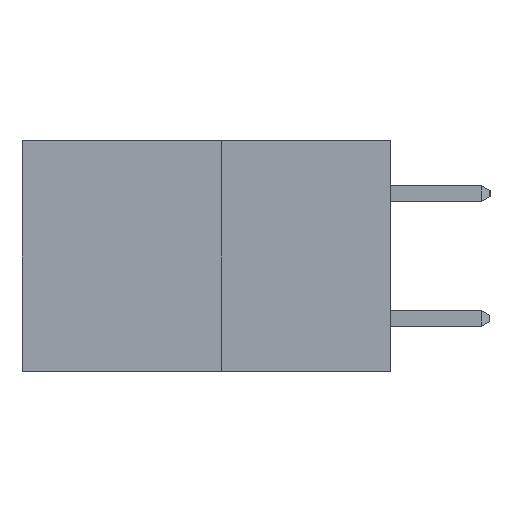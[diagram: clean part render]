
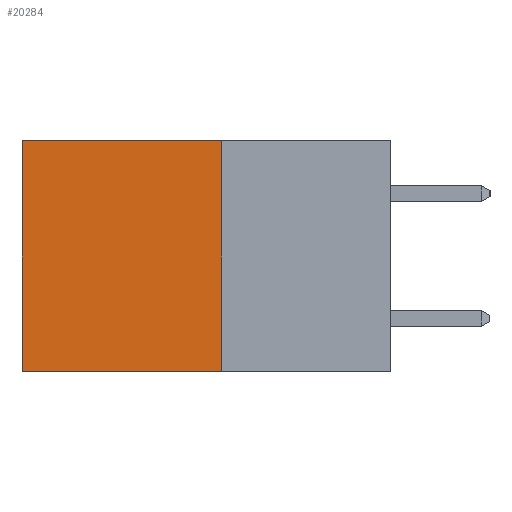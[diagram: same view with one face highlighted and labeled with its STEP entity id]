
A CAD part, left-side view. The second image highlights one B-rep face of the part: STEP entity #20284.
In plain terms, the highlighted planar face has unit normal (-1, 0, 0).
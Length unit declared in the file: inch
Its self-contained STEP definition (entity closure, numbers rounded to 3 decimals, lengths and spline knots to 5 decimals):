
#7 = CARTESIAN_POINT ( 'NONE',  ( 0.277, 0.59, 0. ) ) ;
#1687 = EDGE_CURVE ( 'NONE', #20280, #17652, #16281, .T. ) ;
#2284 = DIRECTION ( 'NONE',  ( 0., 0., -1. ) ) ;
#3063 = PLANE ( 'NONE',  #10664 ) ;
#3429 = VECTOR ( 'NONE', #18031, 39.37008 ) ;
#5241 = ORIENTED_EDGE ( 'NONE', *, *, #1687, .T. ) ;
#5421 = CARTESIAN_POINT ( 'NONE',  ( 0.277, 0.27, 0. ) ) ;
#6672 = DIRECTION ( 'NONE',  ( 1., 0., 0. ) ) ;
#7388 = LINE ( 'NONE', #18371, #21041 ) ;
#7686 = CARTESIAN_POINT ( 'NONE',  ( 0.277, 0.27, -0.37 ) ) ;
#7774 = VECTOR ( 'NONE', #11255, 39.37008 ) ;
#8145 = LINE ( 'NONE', #17963, #3429 ) ;
#9815 = EDGE_CURVE ( 'NONE', #20280, #19087, #7388, .T. ) ;
#9891 = DIRECTION ( 'NONE',  ( 0., 1., 0. ) ) ;
#10664 = AXIS2_PLACEMENT_3D ( 'NONE', #15547, #6672, #19066 ) ;
#11255 = DIRECTION ( 'NONE',  ( 0., 1., 0. ) ) ;
#12172 = ORIENTED_EDGE ( 'NONE', *, *, #18432, .T. ) ;
#12763 = CARTESIAN_POINT ( 'NONE',  ( 0.277, 0.27, -0.37 ) ) ;
#13868 = EDGE_LOOP ( 'NONE', ( #12172, #22288, #17296, #5241 ) ) ;
#15547 = CARTESIAN_POINT ( 'NONE',  ( 0.277, 0.27, -0.37 ) ) ;
#15750 = EDGE_CURVE ( 'NONE', #19087, #20643, #18381, .T. ) ;
#16281 = LINE ( 'NONE', #5421, #20864 ) ;
#17296 = ORIENTED_EDGE ( 'NONE', *, *, #9815, .F. ) ;
#17652 = VERTEX_POINT ( 'NONE', #7 ) ;
#17963 = CARTESIAN_POINT ( 'NONE',  ( 0.277, 0.59, -0.37 ) ) ;
#18031 = DIRECTION ( 'NONE',  ( 0., 0., -1. ) ) ;
#18371 = CARTESIAN_POINT ( 'NONE',  ( 0.277, 0.27, -0.37 ) ) ;
#18381 = LINE ( 'NONE', #7686, #7774 ) ;
#18432 = EDGE_CURVE ( 'NONE', #17652, #20643, #8145, .T. ) ;
#19066 = DIRECTION ( 'NONE',  ( 0., 0., -1. ) ) ;
#19087 = VERTEX_POINT ( 'NONE', #12763 ) ;
#19195 = FACE_OUTER_BOUND ( 'NONE', #13868, .T. ) ;
#19940 = CARTESIAN_POINT ( 'NONE',  ( 0.277, 0.59, -0.37 ) ) ;
#20280 = VERTEX_POINT ( 'NONE', #22368 ) ;
#20284 = ADVANCED_FACE ( 'NONE', ( #19195 ), #3063, .F. ) ;
#20643 = VERTEX_POINT ( 'NONE', #19940 ) ;
#20864 = VECTOR ( 'NONE', #9891, 39.37008 ) ;
#21041 = VECTOR ( 'NONE', #2284, 39.37008 ) ;
#22288 = ORIENTED_EDGE ( 'NONE', *, *, #15750, .F. ) ;
#22368 = CARTESIAN_POINT ( 'NONE',  ( 0.277, 0.27, 0. ) ) ;
